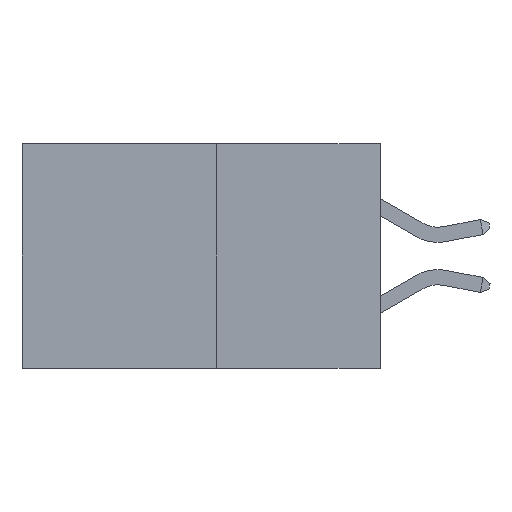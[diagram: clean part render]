
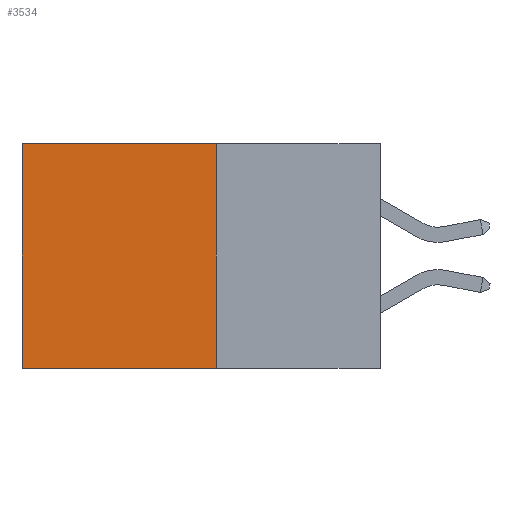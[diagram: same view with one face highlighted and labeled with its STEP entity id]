
A CAD part, left-side view. The second image highlights one B-rep face of the part: STEP entity #3534.
In plain terms, the highlighted planar face has unit normal (-1, 0, 0).
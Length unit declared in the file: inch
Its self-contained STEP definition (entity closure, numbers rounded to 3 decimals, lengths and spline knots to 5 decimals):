
#190 = FACE_OUTER_BOUND ( 'NONE', #2560, .T. ) ;
#1004 = VECTOR ( 'NONE', #3728, 39.37008 ) ;
#1026 = VERTEX_POINT ( 'NONE', #4291 ) ;
#1271 = LINE ( 'NONE', #5874, #8566 ) ;
#1638 = EDGE_CURVE ( 'NONE', #2643, #1026, #1271, .T. ) ;
#2158 = CARTESIAN_POINT ( 'NONE',  ( 0.277, 0.27, 0. ) ) ;
#2560 = EDGE_LOOP ( 'NONE', ( #6794, #8565, #3239, #5199 ) ) ;
#2643 = VERTEX_POINT ( 'NONE', #2158 ) ;
#2850 = DIRECTION ( 'NONE',  ( 0., 0., -1. ) ) ;
#3229 = PLANE ( 'NONE',  #7320 ) ;
#3239 = ORIENTED_EDGE ( 'NONE', *, *, #1638, .F. ) ;
#3250 = DIRECTION ( 'NONE',  ( 1., 0., 0. ) ) ;
#3265 = CARTESIAN_POINT ( 'NONE',  ( 0.277, 0.27, -0.37 ) ) ;
#3534 = ADVANCED_FACE ( 'NONE', ( #190 ), #3229, .F. ) ;
#3728 = DIRECTION ( 'NONE',  ( 0., 1., 0. ) ) ;
#3782 = VERTEX_POINT ( 'NONE', #8323 ) ;
#3919 = LINE ( 'NONE', #5834, #7395 ) ;
#4291 = CARTESIAN_POINT ( 'NONE',  ( 0.277, 0.27, -0.37 ) ) ;
#4295 = EDGE_CURVE ( 'NONE', #3782, #9017, #3919, .T. ) ;
#4441 = CARTESIAN_POINT ( 'NONE',  ( 0.277, 0.27, -0.37 ) ) ;
#4473 = DIRECTION ( 'NONE',  ( 0., 0., -1. ) ) ;
#5199 = ORIENTED_EDGE ( 'NONE', *, *, #6657, .T. ) ;
#5721 = CARTESIAN_POINT ( 'NONE',  ( 0.277, 0.59, -0.37 ) ) ;
#5727 = LINE ( 'NONE', #7911, #8842 ) ;
#5785 = DIRECTION ( 'NONE',  ( 0., 0., -1. ) ) ;
#5834 = CARTESIAN_POINT ( 'NONE',  ( 0.277, 0.59, -0.37 ) ) ;
#5874 = CARTESIAN_POINT ( 'NONE',  ( 0.277, 0.27, -0.37 ) ) ;
#6584 = DIRECTION ( 'NONE',  ( 0., 1., 0. ) ) ;
#6657 = EDGE_CURVE ( 'NONE', #2643, #3782, #5727, .T. ) ;
#6794 = ORIENTED_EDGE ( 'NONE', *, *, #4295, .T. ) ;
#7320 = AXIS2_PLACEMENT_3D ( 'NONE', #3265, #3250, #2850 ) ;
#7395 = VECTOR ( 'NONE', #5785, 39.37008 ) ;
#7530 = EDGE_CURVE ( 'NONE', #1026, #9017, #8724, .T. ) ;
#7911 = CARTESIAN_POINT ( 'NONE',  ( 0.277, 0.27, 0. ) ) ;
#8323 = CARTESIAN_POINT ( 'NONE',  ( 0.277, 0.59, 0. ) ) ;
#8565 = ORIENTED_EDGE ( 'NONE', *, *, #7530, .F. ) ;
#8566 = VECTOR ( 'NONE', #4473, 39.37008 ) ;
#8724 = LINE ( 'NONE', #4441, #1004 ) ;
#8842 = VECTOR ( 'NONE', #6584, 39.37008 ) ;
#9017 = VERTEX_POINT ( 'NONE', #5721 ) ;
